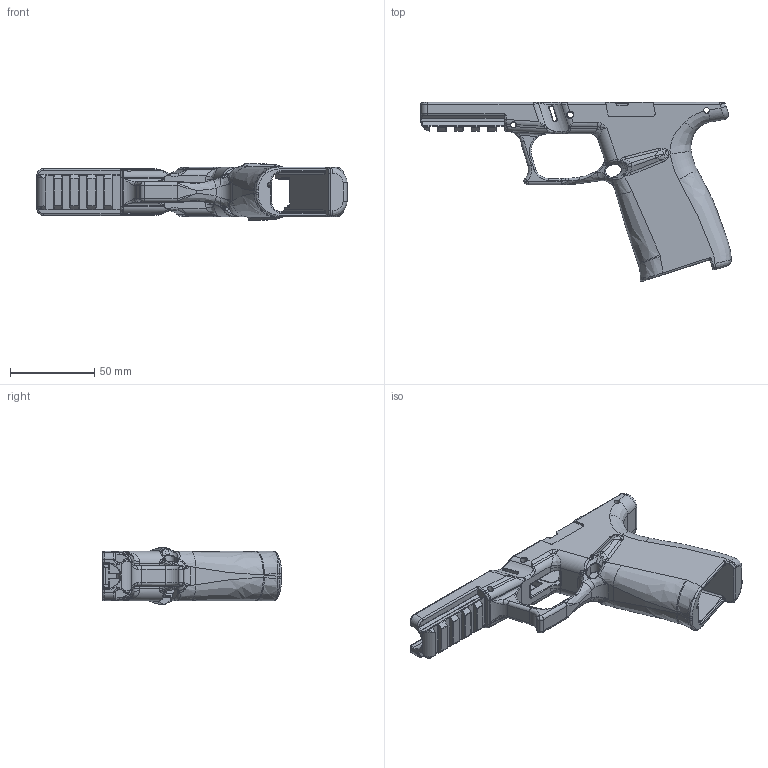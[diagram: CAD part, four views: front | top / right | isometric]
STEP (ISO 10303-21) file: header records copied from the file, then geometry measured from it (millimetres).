
FILE_DESCRIPTION(/* description */ (''),/* implementation_level */ '2;1');
FILE_NAME(/* name */ 'SD40_Carbon Cobra_011522.stp',/* time_stamp */ '2022-01-15T17:31:07-05:00',/* author */ (''),/* organization */ (''),/* preprocessor_version */ 'ST-DEVELOPER v16.7',/* originating_system */ 'SIEMENS PLM Software NX 1899',/* authorisation */ '');
FILE_SCHEMA (('AUTOMOTIVE_DESIGN { 1 0 10303 214 3 1 1 1 }'));
Length unit declared in the file: millimetre
Products named in the file (1): tyle19C8C564rfq8
Bounding box: 183.68 x 105.98 x 34.02 mm (x, y, z)
Volume: 95525.1 mm3; surface area: 45717.5 mm2
Topology: 1 solids, 1 shells, 1461 faces, 3535 edges, 1972 vertices
Faces by surface type: cylinder 516, bspline 512, plane 210, torus 178, cone 26, sphere 18, extrusion 1
Full cylindrical faces by diameter (mm): 2.159 x1, 2.5 x1, 3.175 x2, 3.3 x2, 3.6 x2
Entity records: 56858 total; most frequent: CARTESIAN_POINT 26956, ORIENTED_EDGE 6866, DIRECTION 5369, EDGE_CURVE 3433, AXIS2_PLACEMENT_3D 2151, VERTEX_POINT 1964, EDGE_LOOP 1473, ADVANCED_FACE 1458
